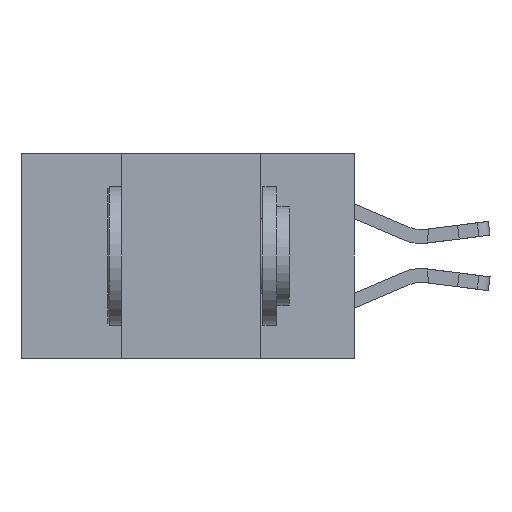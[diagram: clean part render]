
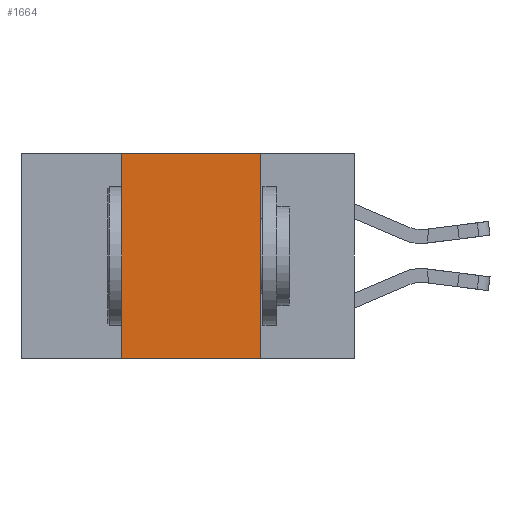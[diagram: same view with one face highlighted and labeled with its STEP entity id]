
A CAD part, left-side view. The second image highlights one B-rep face of the part: STEP entity #1664.
In plain terms, the highlighted planar face has unit normal (-1, 0, 0).
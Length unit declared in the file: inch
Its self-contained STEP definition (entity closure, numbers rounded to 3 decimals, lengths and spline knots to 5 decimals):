
#160 = VECTOR ( 'NONE', #16629, 39.37008 ) ;
#915 = ORIENTED_EDGE ( 'NONE', *, *, #18441, .F. ) ;
#1664 = ADVANCED_FACE ( 'NONE', ( #2694 ), #3898, .F. ) ;
#1794 = AXIS2_PLACEMENT_3D ( 'NONE', #4086, #8787, #8431 ) ;
#1956 = VERTEX_POINT ( 'NONE', #15529 ) ;
#2221 = LINE ( 'NONE', #5232, #10125 ) ;
#2694 = FACE_OUTER_BOUND ( 'NONE', #18607, .T. ) ;
#3601 = ORIENTED_EDGE ( 'NONE', *, *, #13742, .F. ) ;
#3898 = PLANE ( 'NONE',  #1794 ) ;
#4086 = CARTESIAN_POINT ( 'NONE',  ( 0., 0.6, 0. ) ) ;
#4319 = DIRECTION ( 'NONE',  ( 0., -1., 0. ) ) ;
#5232 = CARTESIAN_POINT ( 'NONE',  ( 0., 0.42, -0.37 ) ) ;
#6195 = LINE ( 'NONE', #18996, #18365 ) ;
#6389 = CARTESIAN_POINT ( 'NONE',  ( 0., 0.17, -0.37 ) ) ;
#6805 = DIRECTION ( 'NONE',  ( 0., 0., 1. ) ) ;
#7124 = CARTESIAN_POINT ( 'NONE',  ( 0., 0.42, -0.37 ) ) ;
#7323 = ORIENTED_EDGE ( 'NONE', *, *, #16897, .F. ) ;
#8166 = EDGE_CURVE ( 'NONE', #11770, #16044, #18915, .T. ) ;
#8431 = DIRECTION ( 'NONE',  ( 0., 0., -1. ) ) ;
#8787 = DIRECTION ( 'NONE',  ( 1., 0., 0. ) ) ;
#9063 = CARTESIAN_POINT ( 'NONE',  ( 0., 0.17, 0. ) ) ;
#9307 = ORIENTED_EDGE ( 'NONE', *, *, #8166, .T. ) ;
#10125 = VECTOR ( 'NONE', #6805, 39.37008 ) ;
#11770 = VERTEX_POINT ( 'NONE', #7124 ) ;
#11924 = VERTEX_POINT ( 'NONE', #9063 ) ;
#12678 = DIRECTION ( 'NONE',  ( 0., 0., -1. ) ) ;
#13742 = EDGE_CURVE ( 'NONE', #1956, #11924, #20161, .T. ) ;
#13892 = CARTESIAN_POINT ( 'NONE',  ( 0., 0.6, -0.37 ) ) ;
#14755 = VECTOR ( 'NONE', #4319, 39.37008 ) ;
#15063 = CARTESIAN_POINT ( 'NONE',  ( 0., 0.6, 0. ) ) ;
#15529 = CARTESIAN_POINT ( 'NONE',  ( 0., 0.42, 0. ) ) ;
#16044 = VERTEX_POINT ( 'NONE', #6389 ) ;
#16629 = DIRECTION ( 'NONE',  ( 0., -1., 0. ) ) ;
#16897 = EDGE_CURVE ( 'NONE', #11924, #16044, #6195, .T. ) ;
#18365 = VECTOR ( 'NONE', #12678, 39.37008 ) ;
#18441 = EDGE_CURVE ( 'NONE', #11770, #1956, #2221, .T. ) ;
#18607 = EDGE_LOOP ( 'NONE', ( #7323, #3601, #915, #9307 ) ) ;
#18915 = LINE ( 'NONE', #13892, #14755 ) ;
#18996 = CARTESIAN_POINT ( 'NONE',  ( 0., 0.17, -0.37 ) ) ;
#20161 = LINE ( 'NONE', #15063, #160 ) ;
